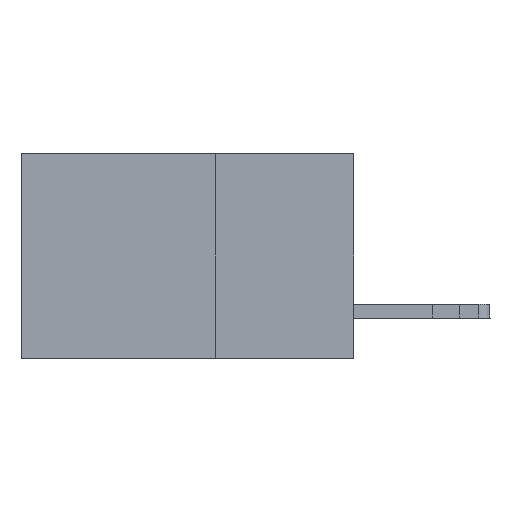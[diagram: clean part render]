
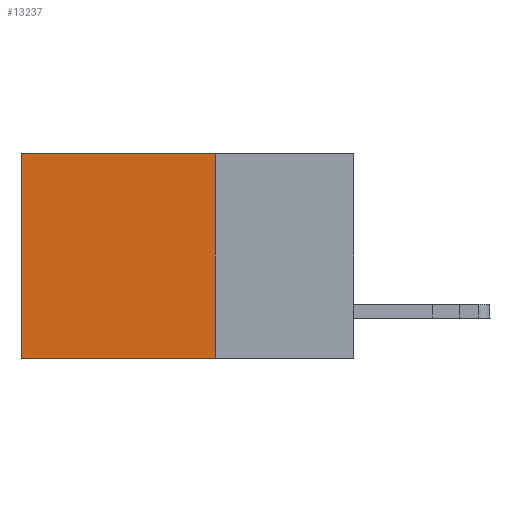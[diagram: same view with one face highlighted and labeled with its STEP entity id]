
A CAD part, left-side view. The second image highlights one B-rep face of the part: STEP entity #13237.
In plain terms, the highlighted planar face has unit normal (-1, 0, 0).
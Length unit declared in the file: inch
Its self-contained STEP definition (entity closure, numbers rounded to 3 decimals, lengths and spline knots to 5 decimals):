
#107 = LINE ( 'NONE', #5836, #17707 ) ;
#114 = PLANE ( 'NONE',  #20113 ) ;
#1114 = EDGE_LOOP ( 'NONE', ( #9809, #21830, #5770, #16980 ) ) ;
#1567 = CARTESIAN_POINT ( 'NONE',  ( 0.2875, 0.6, 0. ) ) ;
#1907 = EDGE_CURVE ( 'NONE', #8766, #2323, #107, .T. ) ;
#2323 = VERTEX_POINT ( 'NONE', #4152 ) ;
#3017 = LINE ( 'NONE', #8467, #6338 ) ;
#3253 = LINE ( 'NONE', #7060, #6985 ) ;
#3500 = EDGE_CURVE ( 'NONE', #6507, #14979, #3017, .T. ) ;
#3818 = DIRECTION ( 'NONE',  ( 1., 0., 0. ) ) ;
#4152 = CARTESIAN_POINT ( 'NONE',  ( 0.2875, 0.6, -0.37 ) ) ;
#4911 = CARTESIAN_POINT ( 'NONE',  ( 0.2875, 0.25, 0. ) ) ;
#5770 = ORIENTED_EDGE ( 'NONE', *, *, #3500, .F. ) ;
#5836 = CARTESIAN_POINT ( 'NONE',  ( 0.2875, 0.6, 0. ) ) ;
#6338 = VECTOR ( 'NONE', #17191, 39.37008 ) ;
#6507 = VERTEX_POINT ( 'NONE', #4911 ) ;
#6985 = VECTOR ( 'NONE', #21446, 39.37008 ) ;
#7060 = CARTESIAN_POINT ( 'NONE',  ( 0.2875, 0.25, 0. ) ) ;
#7376 = DIRECTION ( 'NONE',  ( 0., 0., -1. ) ) ;
#7855 = LINE ( 'NONE', #17255, #19364 ) ;
#8467 = CARTESIAN_POINT ( 'NONE',  ( 0.2875, 0.25, 0. ) ) ;
#8766 = VERTEX_POINT ( 'NONE', #1567 ) ;
#9399 = FACE_OUTER_BOUND ( 'NONE', #1114, .T. ) ;
#9809 = ORIENTED_EDGE ( 'NONE', *, *, #1907, .T. ) ;
#13237 = ADVANCED_FACE ( 'NONE', ( #9399 ), #114, .F. ) ;
#13308 = EDGE_CURVE ( 'NONE', #14979, #2323, #7855, .T. ) ;
#13783 = CARTESIAN_POINT ( 'NONE',  ( 0.2875, 0.25, -0.37 ) ) ;
#14776 = CARTESIAN_POINT ( 'NONE',  ( 0.2875, 0.25, 0. ) ) ;
#14979 = VERTEX_POINT ( 'NONE', #13783 ) ;
#16980 = ORIENTED_EDGE ( 'NONE', *, *, #22680, .T. ) ;
#17191 = DIRECTION ( 'NONE',  ( 0., 0., -1. ) ) ;
#17255 = CARTESIAN_POINT ( 'NONE',  ( 0.2875, 0.25, -0.37 ) ) ;
#17707 = VECTOR ( 'NONE', #18214, 39.37008 ) ;
#18214 = DIRECTION ( 'NONE',  ( 0., 0., -1. ) ) ;
#19364 = VECTOR ( 'NONE', #22608, 39.37008 ) ;
#20113 = AXIS2_PLACEMENT_3D ( 'NONE', #14776, #3818, #7376 ) ;
#21446 = DIRECTION ( 'NONE',  ( 0., 1., 0. ) ) ;
#21830 = ORIENTED_EDGE ( 'NONE', *, *, #13308, .F. ) ;
#22608 = DIRECTION ( 'NONE',  ( 0., 1., 0. ) ) ;
#22680 = EDGE_CURVE ( 'NONE', #6507, #8766, #3253, .T. ) ;
